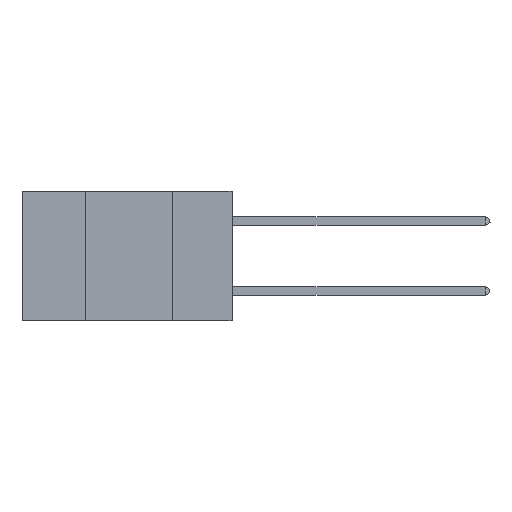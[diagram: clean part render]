
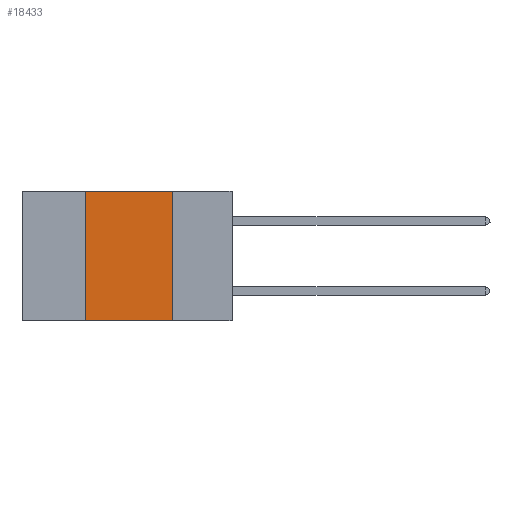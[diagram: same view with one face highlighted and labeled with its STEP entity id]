
A CAD part, left-side view. The second image highlights one B-rep face of the part: STEP entity #18433.
In plain terms, the highlighted planar face has unit normal (-1, 0, 0).
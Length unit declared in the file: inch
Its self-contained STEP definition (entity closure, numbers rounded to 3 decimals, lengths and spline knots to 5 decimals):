
#273 = PLANE ( 'NONE',  #24385 ) ;
#1917 = VECTOR ( 'NONE', #32189, 39.37008 ) ;
#3042 = LINE ( 'NONE', #16615, #7687 ) ;
#4832 = CARTESIAN_POINT ( 'NONE',  ( 0., 0.17, 0. ) ) ;
#6251 = DIRECTION ( 'NONE',  ( 0., 0., -1. ) ) ;
#6381 = CARTESIAN_POINT ( 'NONE',  ( 0., 0.6, 0. ) ) ;
#7687 = VECTOR ( 'NONE', #28240, 39.37008 ) ;
#8280 = DIRECTION ( 'NONE',  ( 0., -1., 0. ) ) ;
#8393 = CARTESIAN_POINT ( 'NONE',  ( 0., 0.42, -0.37 ) ) ;
#8937 = CARTESIAN_POINT ( 'NONE',  ( 0., 0.17, 0. ) ) ;
#9962 = LINE ( 'NONE', #4832, #1917 ) ;
#10916 = VERTEX_POINT ( 'NONE', #8393 ) ;
#12828 = ORIENTED_EDGE ( 'NONE', *, *, #24319, .F. ) ;
#15253 = ORIENTED_EDGE ( 'NONE', *, *, #27273, .F. ) ;
#15403 = EDGE_CURVE ( 'NONE', #10916, #22448, #21667, .T. ) ;
#16190 = ORIENTED_EDGE ( 'NONE', *, *, #22706, .F. ) ;
#16615 = CARTESIAN_POINT ( 'NONE',  ( 0., 0.42, 0. ) ) ;
#18055 = CARTESIAN_POINT ( 'NONE',  ( 0., 0.17, -0.37 ) ) ;
#18433 = ADVANCED_FACE ( 'NONE', ( #22120 ), #273, .F. ) ;
#19298 = CARTESIAN_POINT ( 'NONE',  ( 0., 0.6, 0. ) ) ;
#19467 = DIRECTION ( 'NONE',  ( 1., 0., 0. ) ) ;
#20313 = CARTESIAN_POINT ( 'NONE',  ( 0., 0.42, 0. ) ) ;
#20504 = VERTEX_POINT ( 'NONE', #8937 ) ;
#21667 = LINE ( 'NONE', #32452, #22625 ) ;
#22120 = FACE_OUTER_BOUND ( 'NONE', #23435, .T. ) ;
#22448 = VERTEX_POINT ( 'NONE', #18055 ) ;
#22625 = VECTOR ( 'NONE', #8280, 39.37008 ) ;
#22706 = EDGE_CURVE ( 'NONE', #30019, #20504, #22944, .T. ) ;
#22933 = ORIENTED_EDGE ( 'NONE', *, *, #15403, .T. ) ;
#22944 = LINE ( 'NONE', #6381, #34740 ) ;
#23435 = EDGE_LOOP ( 'NONE', ( #15253, #16190, #12828, #22933 ) ) ;
#24319 = EDGE_CURVE ( 'NONE', #10916, #30019, #3042, .T. ) ;
#24385 = AXIS2_PLACEMENT_3D ( 'NONE', #19298, #19467, #6251 ) ;
#25583 = DIRECTION ( 'NONE',  ( 0., -1., 0. ) ) ;
#27273 = EDGE_CURVE ( 'NONE', #20504, #22448, #9962, .T. ) ;
#28240 = DIRECTION ( 'NONE',  ( 0., 0., 1. ) ) ;
#30019 = VERTEX_POINT ( 'NONE', #20313 ) ;
#32189 = DIRECTION ( 'NONE',  ( 0., 0., -1. ) ) ;
#32452 = CARTESIAN_POINT ( 'NONE',  ( 0., 0.6, -0.37 ) ) ;
#34740 = VECTOR ( 'NONE', #25583, 39.37008 ) ;
